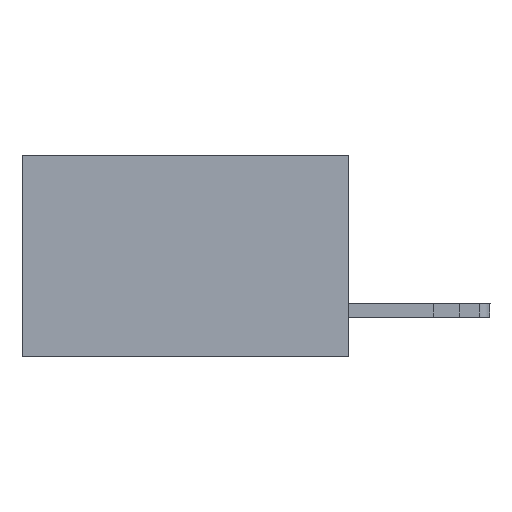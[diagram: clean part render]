
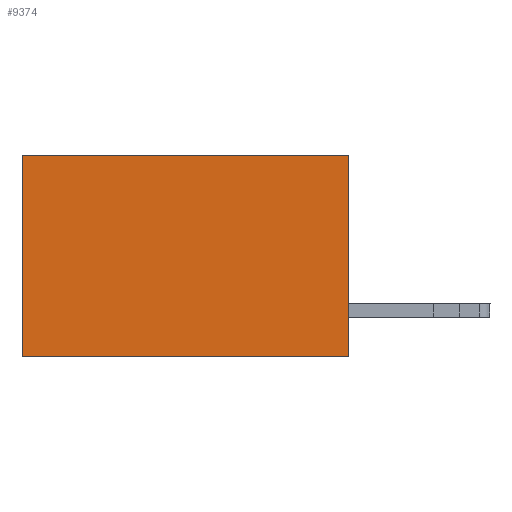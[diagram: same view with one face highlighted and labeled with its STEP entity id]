
A CAD part, left-side view. The second image highlights one B-rep face of the part: STEP entity #9374.
In plain terms, the highlighted planar face has unit normal (-1, 0, 0).
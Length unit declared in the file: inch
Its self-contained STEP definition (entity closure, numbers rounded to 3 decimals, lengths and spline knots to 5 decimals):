
#1298 = EDGE_CURVE ( 'NONE', #5217, #2450, #6541, .T. ) ;
#1515 = EDGE_CURVE ( 'NONE', #2450, #6219, #16069, .T. ) ;
#2065 = ORIENTED_EDGE ( 'NONE', *, *, #11410, .T. ) ;
#2450 = VERTEX_POINT ( 'NONE', #5656 ) ;
#2726 = VECTOR ( 'NONE', #9369, 39.37008 ) ;
#2861 = LINE ( 'NONE', #13137, #9218 ) ;
#3025 = PLANE ( 'NONE',  #3294 ) ;
#3172 = LINE ( 'NONE', #9433, #9509 ) ;
#3248 = VERTEX_POINT ( 'NONE', #4279 ) ;
#3294 = AXIS2_PLACEMENT_3D ( 'NONE', #6845, #4339, #13051 ) ;
#4279 = CARTESIAN_POINT ( 'NONE',  ( 0.2615, 0.6, 0. ) ) ;
#4339 = DIRECTION ( 'NONE',  ( 1., 0., 0. ) ) ;
#4429 = DIRECTION ( 'NONE',  ( 0., 0., -1. ) ) ;
#5217 = VERTEX_POINT ( 'NONE', #7912 ) ;
#5363 = ORIENTED_EDGE ( 'NONE', *, *, #14434, .T. ) ;
#5656 = CARTESIAN_POINT ( 'NONE',  ( 0.2615, 0., -0.37 ) ) ;
#6219 = VERTEX_POINT ( 'NONE', #6519 ) ;
#6335 = VECTOR ( 'NONE', #14730, 39.37008 ) ;
#6519 = CARTESIAN_POINT ( 'NONE',  ( 0.2615, 0.6, -0.37 ) ) ;
#6541 = LINE ( 'NONE', #8346, #2726 ) ;
#6845 = CARTESIAN_POINT ( 'NONE',  ( 0.2615, 0., -0.37 ) ) ;
#7912 = CARTESIAN_POINT ( 'NONE',  ( 0.2615, 0., 0. ) ) ;
#8346 = CARTESIAN_POINT ( 'NONE',  ( 0.2615, 0., -0.37 ) ) ;
#8530 = FACE_OUTER_BOUND ( 'NONE', #9804, .T. ) ;
#9218 = VECTOR ( 'NONE', #4429, 39.37008 ) ;
#9369 = DIRECTION ( 'NONE',  ( 0., 0., -1. ) ) ;
#9374 = ADVANCED_FACE ( 'NONE', ( #8530 ), #3025, .F. ) ;
#9433 = CARTESIAN_POINT ( 'NONE',  ( 0.2615, 0., 0. ) ) ;
#9509 = VECTOR ( 'NONE', #11953, 39.37008 ) ;
#9689 = ORIENTED_EDGE ( 'NONE', *, *, #1515, .F. ) ;
#9804 = EDGE_LOOP ( 'NONE', ( #2065, #9689, #9952, #5363 ) ) ;
#9952 = ORIENTED_EDGE ( 'NONE', *, *, #1298, .F. ) ;
#11410 = EDGE_CURVE ( 'NONE', #3248, #6219, #2861, .T. ) ;
#11953 = DIRECTION ( 'NONE',  ( 0., 1., 0. ) ) ;
#12261 = CARTESIAN_POINT ( 'NONE',  ( 0.2615, 0., -0.37 ) ) ;
#13051 = DIRECTION ( 'NONE',  ( 0., 0., -1. ) ) ;
#13137 = CARTESIAN_POINT ( 'NONE',  ( 0.2615, 0.6, -0.37 ) ) ;
#14434 = EDGE_CURVE ( 'NONE', #5217, #3248, #3172, .T. ) ;
#14730 = DIRECTION ( 'NONE',  ( 0., 1., 0. ) ) ;
#16069 = LINE ( 'NONE', #12261, #6335 ) ;
